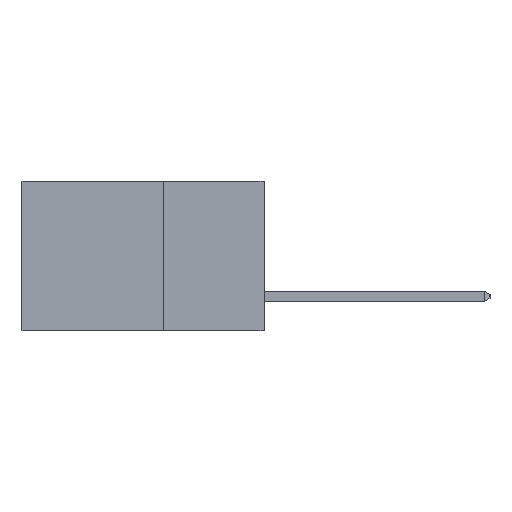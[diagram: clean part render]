
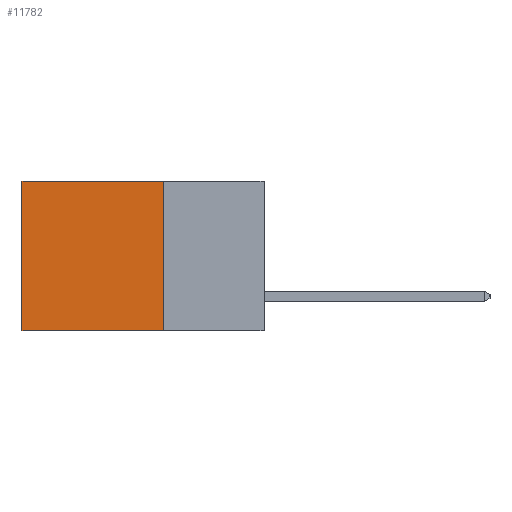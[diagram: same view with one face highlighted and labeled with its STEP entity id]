
A CAD part, left-side view. The second image highlights one B-rep face of the part: STEP entity #11782.
In plain terms, the highlighted planar face has unit normal (-1, 0, 0).
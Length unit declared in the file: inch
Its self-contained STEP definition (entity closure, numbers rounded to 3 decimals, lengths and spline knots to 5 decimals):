
#94 = ORIENTED_EDGE ( 'NONE', *, *, #3995, .T. ) ;
#165 = CARTESIAN_POINT ( 'NONE',  ( 0.298, 0.25, 0. ) ) ;
#220 = DIRECTION ( 'NONE',  ( 0., 0., -1. ) ) ;
#477 = DIRECTION ( 'NONE',  ( 0., 1., 0. ) ) ;
#1310 = CARTESIAN_POINT ( 'NONE',  ( 0.298, 0.6, 0. ) ) ;
#1630 = CARTESIAN_POINT ( 'NONE',  ( 0.298, 0.25, -0.37 ) ) ;
#2008 = VECTOR ( 'NONE', #477, 39.37008 ) ;
#2306 = ORIENTED_EDGE ( 'NONE', *, *, #4993, .F. ) ;
#2447 = VECTOR ( 'NONE', #7940, 39.37008 ) ;
#2536 = EDGE_CURVE ( 'NONE', #11222, #11720, #4742, .T. ) ;
#3173 = CARTESIAN_POINT ( 'NONE',  ( 0.298, 0.25, -0.37 ) ) ;
#3584 = LINE ( 'NONE', #6078, #10105 ) ;
#3995 = EDGE_CURVE ( 'NONE', #11667, #5818, #6447, .T. ) ;
#4060 = EDGE_LOOP ( 'NONE', ( #4847, #6666, #2306, #94 ) ) ;
#4463 = AXIS2_PLACEMENT_3D ( 'NONE', #10226, #6334, #220 ) ;
#4742 = LINE ( 'NONE', #1630, #2008 ) ;
#4751 = EDGE_CURVE ( 'NONE', #5818, #11720, #10552, .T. ) ;
#4847 = ORIENTED_EDGE ( 'NONE', *, *, #4751, .T. ) ;
#4993 = EDGE_CURVE ( 'NONE', #11667, #11222, #3584, .T. ) ;
#5054 = CARTESIAN_POINT ( 'NONE',  ( 0.298, 0.25, 0. ) ) ;
#5818 = VERTEX_POINT ( 'NONE', #6149 ) ;
#6051 = CARTESIAN_POINT ( 'NONE',  ( 0.298, 0.6, -0.37 ) ) ;
#6078 = CARTESIAN_POINT ( 'NONE',  ( 0.298, 0.25, 0. ) ) ;
#6149 = CARTESIAN_POINT ( 'NONE',  ( 0.298, 0.6, 0. ) ) ;
#6154 = VECTOR ( 'NONE', #7473, 39.37008 ) ;
#6334 = DIRECTION ( 'NONE',  ( 1., 0., 0. ) ) ;
#6447 = LINE ( 'NONE', #165, #6154 ) ;
#6666 = ORIENTED_EDGE ( 'NONE', *, *, #2536, .F. ) ;
#7473 = DIRECTION ( 'NONE',  ( 0., 1., 0. ) ) ;
#7815 = FACE_OUTER_BOUND ( 'NONE', #4060, .T. ) ;
#7940 = DIRECTION ( 'NONE',  ( 0., 0., -1. ) ) ;
#10105 = VECTOR ( 'NONE', #10624, 39.37008 ) ;
#10226 = CARTESIAN_POINT ( 'NONE',  ( 0.298, 0.25, 0. ) ) ;
#10552 = LINE ( 'NONE', #1310, #2447 ) ;
#10624 = DIRECTION ( 'NONE',  ( 0., 0., -1. ) ) ;
#11222 = VERTEX_POINT ( 'NONE', #3173 ) ;
#11667 = VERTEX_POINT ( 'NONE', #5054 ) ;
#11720 = VERTEX_POINT ( 'NONE', #6051 ) ;
#11782 = ADVANCED_FACE ( 'NONE', ( #7815 ), #12138, .F. ) ;
#12138 = PLANE ( 'NONE',  #4463 ) ;
